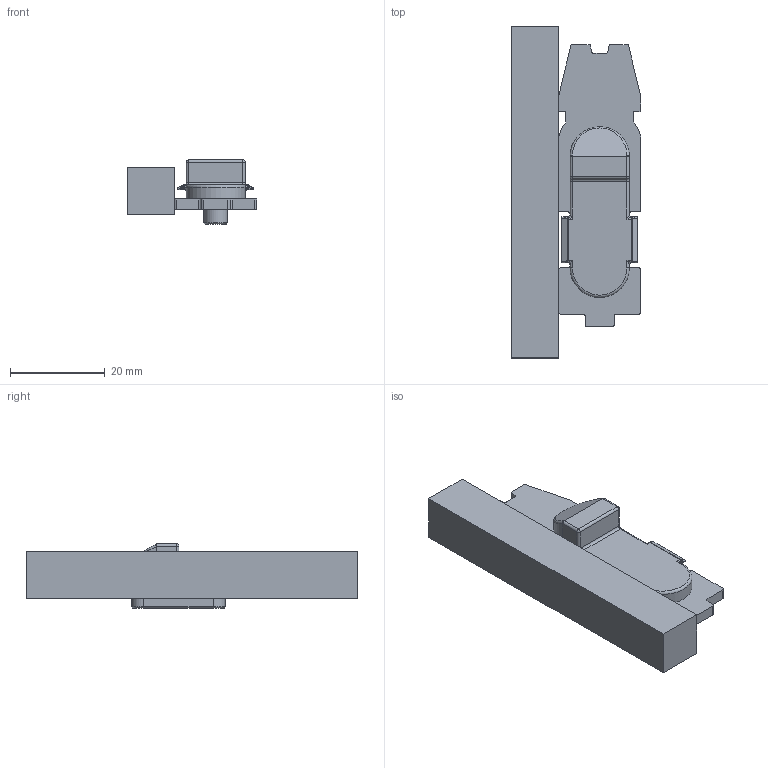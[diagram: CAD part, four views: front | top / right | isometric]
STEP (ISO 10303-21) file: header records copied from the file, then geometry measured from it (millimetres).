
FILE_DESCRIPTION(('FreeCAD Model'),'2;1');
FILE_NAME('Open CASCADE Shape Model','2025-07-14T13:26:58',(''),(''), 'Open CASCADE STEP processor 7.8','FreeCAD','Unknown');
FILE_SCHEMA(('AUTOMOTIVE_DESIGN { 1 0 10303 214 1 1 1 1 }'));
Length unit declared in the file: millimetre
Products named in the file (3): Unnamed; Cut001; Cube002
Assembly tree (2 placements, depth 2):
  Unnamed
    Cut001
    Cube002
Bounding box: 27.4 x 70 x 13.55 mm (x, y, z)
Volume: 11171.2 mm3; surface area: 5789.7 mm2
Topology: 2 solids, 2 shells, 138 faces, 357 edges, 210 vertices
Faces by surface type: plane 57, cylinder 56, bspline 18, torus 3, sphere 2, cone 2
Entity records: 4429 total; most frequent: CARTESIAN_POINT 1244, ORIENTED_EDGE 686, DIRECTION 628, EDGE_CURVE 343, AXIS2_PLACEMENT_3D 210, VERTEX_POINT 210, LINE 208, VECTOR 208
